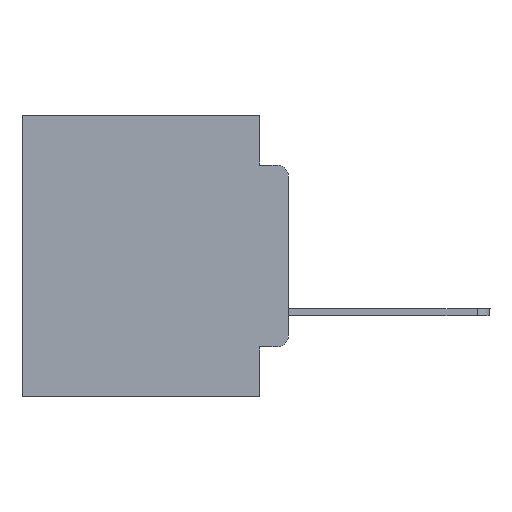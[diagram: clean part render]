
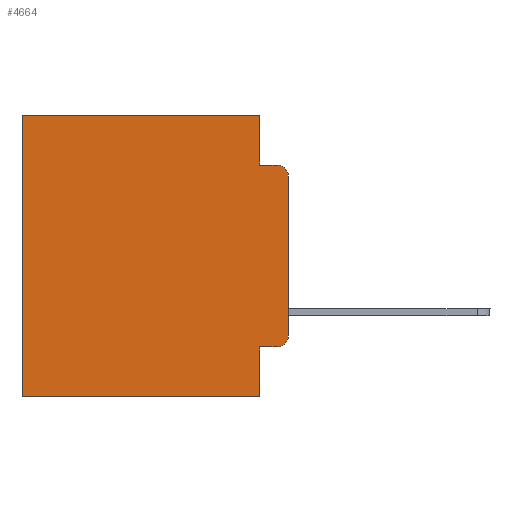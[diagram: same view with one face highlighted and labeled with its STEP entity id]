
A CAD part, left-side view. The second image highlights one B-rep face of the part: STEP entity #4664.
In plain terms, the highlighted planar face has unit normal (-1, 0, 0).
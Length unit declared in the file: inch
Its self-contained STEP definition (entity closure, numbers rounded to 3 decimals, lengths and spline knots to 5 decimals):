
#436 = ORIENTED_EDGE ( 'NONE', *, *, #8709, .T. ) ;
#805 = DIRECTION ( 'NONE',  ( 0., 0., -1. ) ) ;
#890 = CIRCLE ( 'NONE', #15533, 0.02 ) ;
#1123 = DIRECTION ( 'NONE',  ( 0., 0., -1. ) ) ;
#1189 = ORIENTED_EDGE ( 'NONE', *, *, #14981, .T. ) ;
#1551 = CARTESIAN_POINT ( 'NONE',  ( 0.298, 0.051, -0.4115 ) ) ;
#1937 = CARTESIAN_POINT ( 'NONE',  ( 0.298, 0.02, -0.3915 ) ) ;
#2203 = CARTESIAN_POINT ( 'NONE',  ( 0.298, 0., -0.3915 ) ) ;
#2220 = VERTEX_POINT ( 'NONE', #2203 ) ;
#2901 = EDGE_CURVE ( 'NONE', #13639, #3226, #22804, .T. ) ;
#3183 = CARTESIAN_POINT ( 'NONE',  ( 0.298, 0.051, 0. ) ) ;
#3226 = VERTEX_POINT ( 'NONE', #24510 ) ;
#3717 = CARTESIAN_POINT ( 'NONE',  ( 0.298, 0.02, -0.0885 ) ) ;
#4391 = LINE ( 'NONE', #24322, #14721 ) ;
#4428 = AXIS2_PLACEMENT_3D ( 'NONE', #7284, #22326, #805 ) ;
#4514 = DIRECTION ( 'NONE',  ( 0., 0., -1. ) ) ;
#4555 = CARTESIAN_POINT ( 'NONE',  ( 0.298, 0., -0.1085 ) ) ;
#4570 = DIRECTION ( 'NONE',  ( 0., 0., -1. ) ) ;
#4664 = ADVANCED_FACE ( 'NONE', ( #16186 ), #26915, .F. ) ;
#4759 = VERTEX_POINT ( 'NONE', #21155 ) ;
#4787 = DIRECTION ( 'NONE',  ( 0., 0., -1. ) ) ;
#5117 = VECTOR ( 'NONE', #1123, 39.37008 ) ;
#5268 = VECTOR ( 'NONE', #16248, 39.37008 ) ;
#6057 = ORIENTED_EDGE ( 'NONE', *, *, #10540, .F. ) ;
#6631 = CARTESIAN_POINT ( 'NONE',  ( 0.298, 0.473, 0. ) ) ;
#7284 = CARTESIAN_POINT ( 'NONE',  ( 0.298, 0., 0. ) ) ;
#7473 = VECTOR ( 'NONE', #10933, 39.37008 ) ;
#7805 = ORIENTED_EDGE ( 'NONE', *, *, #28178, .F. ) ;
#8481 = CARTESIAN_POINT ( 'NONE',  ( 0.298, 0.051, -0.5 ) ) ;
#8709 = EDGE_CURVE ( 'NONE', #9760, #2220, #890, .T. ) ;
#9079 = ORIENTED_EDGE ( 'NONE', *, *, #14307, .T. ) ;
#9389 = CIRCLE ( 'NONE', #17215, 0.02 ) ;
#9718 = VERTEX_POINT ( 'NONE', #6631 ) ;
#9760 = VERTEX_POINT ( 'NONE', #18079 ) ;
#10540 = EDGE_CURVE ( 'NONE', #26496, #4759, #4391, .T. ) ;
#10791 = ORIENTED_EDGE ( 'NONE', *, *, #19721, .F. ) ;
#10933 = DIRECTION ( 'NONE',  ( 0., -1., 0. ) ) ;
#11766 = CARTESIAN_POINT ( 'NONE',  ( 0.298, 0.051, -0.4115 ) ) ;
#12140 = LINE ( 'NONE', #27588, #15601 ) ;
#12712 = EDGE_CURVE ( 'NONE', #25127, #9760, #22636, .T. ) ;
#13344 = CARTESIAN_POINT ( 'NONE',  ( 0.298, 0.051, 0. ) ) ;
#13639 = VERTEX_POINT ( 'NONE', #18817 ) ;
#13861 = ORIENTED_EDGE ( 'NONE', *, *, #2901, .F. ) ;
#14307 = EDGE_CURVE ( 'NONE', #17781, #21795, #9389, .T. ) ;
#14496 = ORIENTED_EDGE ( 'NONE', *, *, #12712, .T. ) ;
#14721 = VECTOR ( 'NONE', #26465, 39.37008 ) ;
#14981 = EDGE_CURVE ( 'NONE', #13639, #9718, #22153, .T. ) ;
#15533 = AXIS2_PLACEMENT_3D ( 'NONE', #1937, #17430, #4514 ) ;
#15601 = VECTOR ( 'NONE', #16573, 39.37008 ) ;
#15676 = DIRECTION ( 'NONE',  ( -1., 0., 0. ) ) ;
#15821 = DIRECTION ( 'NONE',  ( 0., 0., -1. ) ) ;
#15915 = VECTOR ( 'NONE', #17438, 39.37008 ) ;
#16064 = CARTESIAN_POINT ( 'NONE',  ( 0.298, 0., 0. ) ) ;
#16186 = FACE_OUTER_BOUND ( 'NONE', #25814, .T. ) ;
#16248 = DIRECTION ( 'NONE',  ( 0., 0., -1. ) ) ;
#16573 = DIRECTION ( 'NONE',  ( 0., -1., 0. ) ) ;
#16611 = EDGE_CURVE ( 'NONE', #9718, #4759, #26412, .T. ) ;
#17215 = AXIS2_PLACEMENT_3D ( 'NONE', #24692, #15676, #15821 ) ;
#17430 = DIRECTION ( 'NONE',  ( -1., 0., 0. ) ) ;
#17438 = DIRECTION ( 'NONE',  ( 0., 1., 0. ) ) ;
#17781 = VERTEX_POINT ( 'NONE', #4555 ) ;
#18079 = CARTESIAN_POINT ( 'NONE',  ( 0.298, 0.02, -0.4115 ) ) ;
#18620 = VECTOR ( 'NONE', #4787, 39.37008 ) ;
#18817 = CARTESIAN_POINT ( 'NONE',  ( 0.298, 0.051, 0. ) ) ;
#19536 = CARTESIAN_POINT ( 'NONE',  ( 0.298, 0.473, 0. ) ) ;
#19721 = EDGE_CURVE ( 'NONE', #3226, #21795, #12140, .T. ) ;
#21155 = CARTESIAN_POINT ( 'NONE',  ( 0.298, 0.473, -0.5 ) ) ;
#21795 = VERTEX_POINT ( 'NONE', #3717 ) ;
#22153 = LINE ( 'NONE', #24303, #15915 ) ;
#22326 = DIRECTION ( 'NONE',  ( 1., 0., 0. ) ) ;
#22487 = LINE ( 'NONE', #13344, #25083 ) ;
#22625 = EDGE_CURVE ( 'NONE', #17781, #2220, #26942, .T. ) ;
#22636 = LINE ( 'NONE', #11766, #7473 ) ;
#22707 = ORIENTED_EDGE ( 'NONE', *, *, #16611, .T. ) ;
#22804 = LINE ( 'NONE', #3183, #5268 ) ;
#24303 = CARTESIAN_POINT ( 'NONE',  ( 0.298, 0., 0. ) ) ;
#24322 = CARTESIAN_POINT ( 'NONE',  ( 0.298, 0., -0.5 ) ) ;
#24510 = CARTESIAN_POINT ( 'NONE',  ( 0.298, 0.051, -0.0885 ) ) ;
#24692 = CARTESIAN_POINT ( 'NONE',  ( 0.298, 0.02, -0.1085 ) ) ;
#25083 = VECTOR ( 'NONE', #4570, 39.37008 ) ;
#25127 = VERTEX_POINT ( 'NONE', #1551 ) ;
#25814 = EDGE_LOOP ( 'NONE', ( #26810, #9079, #10791, #13861, #1189, #22707, #6057, #7805, #14496, #436 ) ) ;
#26412 = LINE ( 'NONE', #19536, #18620 ) ;
#26465 = DIRECTION ( 'NONE',  ( 0., 1., 0. ) ) ;
#26496 = VERTEX_POINT ( 'NONE', #8481 ) ;
#26810 = ORIENTED_EDGE ( 'NONE', *, *, #22625, .F. ) ;
#26915 = PLANE ( 'NONE',  #4428 ) ;
#26942 = LINE ( 'NONE', #16064, #5117 ) ;
#27588 = CARTESIAN_POINT ( 'NONE',  ( 0.298, 0.051, -0.0885 ) ) ;
#28178 = EDGE_CURVE ( 'NONE', #25127, #26496, #22487, .T. ) ;
